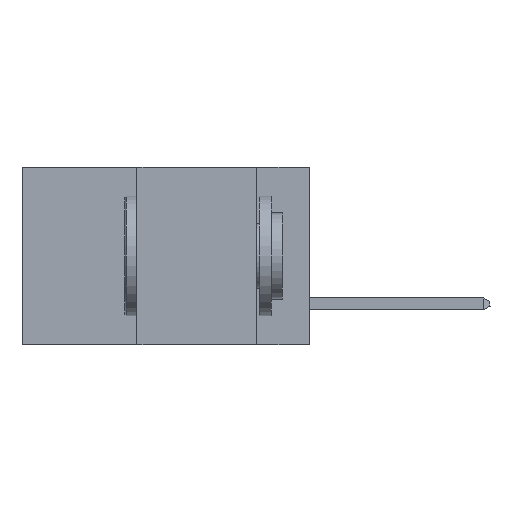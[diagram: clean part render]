
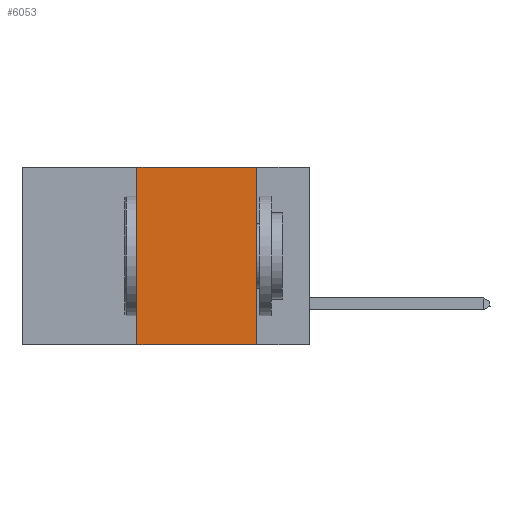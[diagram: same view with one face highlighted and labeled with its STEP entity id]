
A CAD part, left-side view. The second image highlights one B-rep face of the part: STEP entity #6053.
In plain terms, the highlighted planar face has unit normal (-1, 0, 0).
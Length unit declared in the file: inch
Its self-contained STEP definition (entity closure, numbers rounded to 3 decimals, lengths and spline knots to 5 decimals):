
#92 = ORIENTED_EDGE ( 'NONE', *, *, #919, .F. ) ;
#587 = EDGE_CURVE ( 'NONE', #10277, #2500, #10618, .T. ) ;
#919 = EDGE_CURVE ( 'NONE', #7611, #10947, #1785, .T. ) ;
#1241 = DIRECTION ( 'NONE',  ( 1., 0., 0. ) ) ;
#1384 = VECTOR ( 'NONE', #6955, 39.37008 ) ;
#1597 = CARTESIAN_POINT ( 'NONE',  ( 0., 0.6, 0. ) ) ;
#1785 = LINE ( 'NONE', #4323, #9222 ) ;
#2500 = VERTEX_POINT ( 'NONE', #7035 ) ;
#3108 = VECTOR ( 'NONE', #8711, 39.37008 ) ;
#3184 = ORIENTED_EDGE ( 'NONE', *, *, #6967, .F. ) ;
#3244 = EDGE_LOOP ( 'NONE', ( #11307, #3184, #92, #6737 ) ) ;
#3425 = CARTESIAN_POINT ( 'NONE',  ( 0., 0.11, 0. ) ) ;
#3629 = VECTOR ( 'NONE', #10275, 39.37008 ) ;
#3766 = LINE ( 'NONE', #1597, #3629 ) ;
#3822 = PLANE ( 'NONE',  #7742 ) ;
#4323 = CARTESIAN_POINT ( 'NONE',  ( 0., 0.36, 0. ) ) ;
#4334 = EDGE_CURVE ( 'NONE', #7611, #2500, #7799, .T. ) ;
#6053 = ADVANCED_FACE ( 'NONE', ( #9828 ), #3822, .F. ) ;
#6154 = CARTESIAN_POINT ( 'NONE',  ( 0., 0.6, -0.37 ) ) ;
#6247 = CARTESIAN_POINT ( 'NONE',  ( 0., 0.36, -0.37 ) ) ;
#6737 = ORIENTED_EDGE ( 'NONE', *, *, #4334, .T. ) ;
#6741 = CARTESIAN_POINT ( 'NONE',  ( 0., 0.11, 0. ) ) ;
#6955 = DIRECTION ( 'NONE',  ( 0., 0., -1. ) ) ;
#6967 = EDGE_CURVE ( 'NONE', #10947, #10277, #3766, .T. ) ;
#7035 = CARTESIAN_POINT ( 'NONE',  ( 0., 0.11, -0.37 ) ) ;
#7611 = VERTEX_POINT ( 'NONE', #6247 ) ;
#7742 = AXIS2_PLACEMENT_3D ( 'NONE', #9979, #1241, #8096 ) ;
#7799 = LINE ( 'NONE', #6154, #3108 ) ;
#8096 = DIRECTION ( 'NONE',  ( 0., 0., -1. ) ) ;
#8711 = DIRECTION ( 'NONE',  ( 0., -1., 0. ) ) ;
#9222 = VECTOR ( 'NONE', #11242, 39.37008 ) ;
#9828 = FACE_OUTER_BOUND ( 'NONE', #3244, .T. ) ;
#9979 = CARTESIAN_POINT ( 'NONE',  ( 0., 0.6, 0. ) ) ;
#10275 = DIRECTION ( 'NONE',  ( 0., -1., 0. ) ) ;
#10277 = VERTEX_POINT ( 'NONE', #6741 ) ;
#10618 = LINE ( 'NONE', #3425, #1384 ) ;
#10947 = VERTEX_POINT ( 'NONE', #11308 ) ;
#11242 = DIRECTION ( 'NONE',  ( 0., 0., 1. ) ) ;
#11307 = ORIENTED_EDGE ( 'NONE', *, *, #587, .F. ) ;
#11308 = CARTESIAN_POINT ( 'NONE',  ( 0., 0.36, 0. ) ) ;
